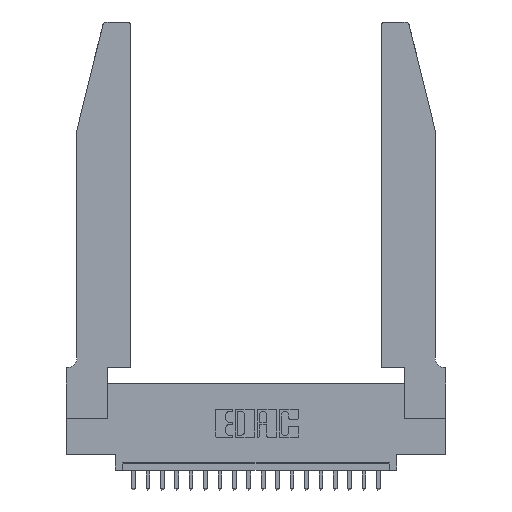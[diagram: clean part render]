
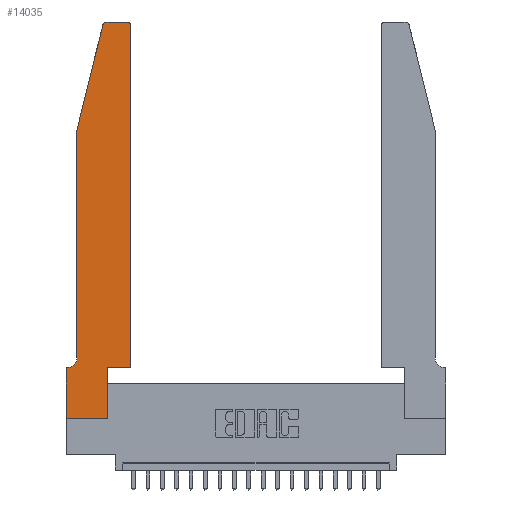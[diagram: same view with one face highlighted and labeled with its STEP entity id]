
A CAD part, top view. The second image highlights one B-rep face of the part: STEP entity #14035.
In plain terms, the highlighted planar face has unit normal (0, 0, 1).
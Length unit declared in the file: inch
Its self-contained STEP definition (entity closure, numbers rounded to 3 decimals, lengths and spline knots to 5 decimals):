
#150 = VERTEX_POINT ( 'NONE', #3158 ) ;
#378 = CARTESIAN_POINT ( 'NONE',  ( 0., 0., 0.37 ) ) ;
#388 = AXIS2_PLACEMENT_3D ( 'NONE', #6410, #19944, #12965 ) ;
#404 = VERTEX_POINT ( 'NONE', #1199 ) ;
#863 = DIRECTION ( 'NONE',  ( -1., 0., 0. ) ) ;
#1165 = LINE ( 'NONE', #7413, #15351 ) ;
#1199 = CARTESIAN_POINT ( 'NONE',  ( 0.25487, 2.72718, 0.37 ) ) ;
#1498 = VERTEX_POINT ( 'NONE', #12572 ) ;
#1550 = VERTEX_POINT ( 'NONE', #11248 ) ;
#1951 = EDGE_CURVE ( 'NONE', #150, #15944, #6328, .T. ) ;
#2256 = EDGE_CURVE ( 'NONE', #1498, #12166, #5822, .T. ) ;
#2539 = CIRCLE ( 'NONE', #16249, 0.03 ) ;
#2664 = DIRECTION ( 'NONE',  ( -1., 0., 0. ) ) ;
#3134 = CARTESIAN_POINT ( 'NONE',  ( 0.2865, 0., 0.37 ) ) ;
#3158 = CARTESIAN_POINT ( 'NONE',  ( 0.0755, 0.42, 0.37 ) ) ;
#3161 = CARTESIAN_POINT ( 'NONE',  ( 0.4505, 0.35, 0.37 ) ) ;
#3423 = DIRECTION ( 'NONE',  ( 0., 1., 0. ) ) ;
#3973 = DIRECTION ( 'NONE',  ( 0., 1., 0. ) ) ;
#4197 = VERTEX_POINT ( 'NONE', #13778 ) ;
#4303 = PLANE ( 'NONE',  #16320 ) ;
#4590 = VERTEX_POINT ( 'NONE', #8246 ) ;
#4596 = EDGE_CURVE ( 'NONE', #1550, #150, #16004, .T. ) ;
#4600 = LINE ( 'NONE', #3161, #20639 ) ;
#4696 = EDGE_LOOP ( 'NONE', ( #13682, #17615, #16482, #18126, #14326, #13669, #9880, #19805, #5662, #19919, #7811, #12443 ) ) ;
#5203 = LINE ( 'NONE', #5921, #19636 ) ;
#5378 = DIRECTION ( 'NONE',  ( 1., 0., 0. ) ) ;
#5662 = ORIENTED_EDGE ( 'NONE', *, *, #7696, .T. ) ;
#5822 = LINE ( 'NONE', #18886, #13185 ) ;
#5921 = CARTESIAN_POINT ( 'NONE',  ( 0.2605, 2.75, 0.37 ) ) ;
#6328 = CIRCLE ( 'NONE', #17832, 0.07 ) ;
#6410 = CARTESIAN_POINT ( 'NONE',  ( 0.284, 2.72, 0.37 ) ) ;
#6680 = VECTOR ( 'NONE', #3973, 39.37008 ) ;
#6788 = DIRECTION ( 'NONE',  ( 0., -1., 0. ) ) ;
#7171 = CARTESIAN_POINT ( 'NONE',  ( 0.4505, 0.35, 0.37 ) ) ;
#7272 = EDGE_CURVE ( 'NONE', #20779, #11202, #4600, .T. ) ;
#7413 = CARTESIAN_POINT ( 'NONE',  ( 0.0755, 0.35, 0.37 ) ) ;
#7421 = DIRECTION ( 'NONE',  ( 0., 0., -1. ) ) ;
#7562 = EDGE_CURVE ( 'NONE', #11202, #4197, #13277, .T. ) ;
#7578 = DIRECTION ( 'NONE',  ( 0., 0., 1. ) ) ;
#7696 = EDGE_CURVE ( 'NONE', #10893, #20779, #12731, .T. ) ;
#7788 = EDGE_CURVE ( 'NONE', #4590, #404, #11410, .T. ) ;
#7811 = ORIENTED_EDGE ( 'NONE', *, *, #7562, .T. ) ;
#8246 = CARTESIAN_POINT ( 'NONE',  ( 0.284, 2.75, 0.37 ) ) ;
#8333 = CARTESIAN_POINT ( 'NONE',  ( 0.0755, 2., 0.37 ) ) ;
#9270 = DIRECTION ( 'NONE',  ( 1., 0., 0. ) ) ;
#9790 = LINE ( 'NONE', #16785, #16121 ) ;
#9880 = ORIENTED_EDGE ( 'NONE', *, *, #2256, .T. ) ;
#9930 = VECTOR ( 'NONE', #6788, 39.37008 ) ;
#10200 = EDGE_CURVE ( 'NONE', #4197, #20260, #2539, .T. ) ;
#10612 = VECTOR ( 'NONE', #3423, 39.37008 ) ;
#10893 = VERTEX_POINT ( 'NONE', #3134 ) ;
#11077 = DIRECTION ( 'NONE',  ( -1., 0., 0. ) ) ;
#11202 = VERTEX_POINT ( 'NONE', #7171 ) ;
#11248 = CARTESIAN_POINT ( 'NONE',  ( 0.0755, 2., 0.37 ) ) ;
#11309 = EDGE_CURVE ( 'NONE', #20260, #4590, #5203, .T. ) ;
#11410 = CIRCLE ( 'NONE', #388, 0.03 ) ;
#12074 = DIRECTION ( 'NONE',  ( 0., 0., 1. ) ) ;
#12166 = VERTEX_POINT ( 'NONE', #378 ) ;
#12443 = ORIENTED_EDGE ( 'NONE', *, *, #10200, .T. ) ;
#12572 = CARTESIAN_POINT ( 'NONE',  ( 0., 0.35, 0.37 ) ) ;
#12582 = EDGE_CURVE ( 'NONE', #404, #1550, #20129, .T. ) ;
#12731 = LINE ( 'NONE', #13953, #6680 ) ;
#12965 = DIRECTION ( 'NONE',  ( 1., 0., 0. ) ) ;
#13081 = CARTESIAN_POINT ( 'NONE',  ( 0.0755, 2., 0.37 ) ) ;
#13185 = VECTOR ( 'NONE', #15936, 39.37008 ) ;
#13256 = FACE_OUTER_BOUND ( 'NONE', #4696, .T. ) ;
#13277 = LINE ( 'NONE', #13437, #10612 ) ;
#13437 = CARTESIAN_POINT ( 'NONE',  ( 0.4505, 0.35, 0.37 ) ) ;
#13669 = ORIENTED_EDGE ( 'NONE', *, *, #17883, .T. ) ;
#13682 = ORIENTED_EDGE ( 'NONE', *, *, #11309, .T. ) ;
#13778 = CARTESIAN_POINT ( 'NONE',  ( 0.4505, 2.72, 0.37 ) ) ;
#13953 = CARTESIAN_POINT ( 'NONE',  ( 0.2865, 0.35, 0.37 ) ) ;
#14035 = ADVANCED_FACE ( 'NONE', ( #13256 ), #4303, .T. ) ;
#14134 = CARTESIAN_POINT ( 'NONE',  ( 0.0055, 0.42, 0.37 ) ) ;
#14292 = EDGE_CURVE ( 'NONE', #12166, #10893, #9790, .T. ) ;
#14326 = ORIENTED_EDGE ( 'NONE', *, *, #1951, .T. ) ;
#15351 = VECTOR ( 'NONE', #11077, 39.37008 ) ;
#15908 = CARTESIAN_POINT ( 'NONE',  ( 0., 0.35, 0.37 ) ) ;
#15936 = DIRECTION ( 'NONE',  ( 0., -1., 0. ) ) ;
#15944 = VERTEX_POINT ( 'NONE', #18100 ) ;
#16004 = LINE ( 'NONE', #8333, #9930 ) ;
#16121 = VECTOR ( 'NONE', #21512, 39.37008 ) ;
#16249 = AXIS2_PLACEMENT_3D ( 'NONE', #20429, #12074, #5378 ) ;
#16320 = AXIS2_PLACEMENT_3D ( 'NONE', #15908, #7578, #9270 ) ;
#16482 = ORIENTED_EDGE ( 'NONE', *, *, #12582, .T. ) ;
#16689 = DIRECTION ( 'NONE',  ( -0.239, -0.971, 0. ) ) ;
#16785 = CARTESIAN_POINT ( 'NONE',  ( 0., 0., 0.37 ) ) ;
#16979 = VECTOR ( 'NONE', #16689, 39.37008 ) ;
#17163 = CARTESIAN_POINT ( 'NONE',  ( 0.2865, 0.35, 0.37 ) ) ;
#17615 = ORIENTED_EDGE ( 'NONE', *, *, #7788, .T. ) ;
#17832 = AXIS2_PLACEMENT_3D ( 'NONE', #14134, #7421, #863 ) ;
#17883 = EDGE_CURVE ( 'NONE', #15944, #1498, #1165, .T. ) ;
#18100 = CARTESIAN_POINT ( 'NONE',  ( 0.0055, 0.35, 0.37 ) ) ;
#18126 = ORIENTED_EDGE ( 'NONE', *, *, #4596, .T. ) ;
#18886 = CARTESIAN_POINT ( 'NONE',  ( 0., 0., 0.37 ) ) ;
#19636 = VECTOR ( 'NONE', #2664, 39.37008 ) ;
#19805 = ORIENTED_EDGE ( 'NONE', *, *, #14292, .T. ) ;
#19919 = ORIENTED_EDGE ( 'NONE', *, *, #7272, .T. ) ;
#19944 = DIRECTION ( 'NONE',  ( 0., 0., 1. ) ) ;
#20129 = LINE ( 'NONE', #13081, #16979 ) ;
#20260 = VERTEX_POINT ( 'NONE', #20302 ) ;
#20302 = CARTESIAN_POINT ( 'NONE',  ( 0.4205, 2.75, 0.37 ) ) ;
#20376 = DIRECTION ( 'NONE',  ( 1., 0., 0. ) ) ;
#20429 = CARTESIAN_POINT ( 'NONE',  ( 0.4205, 2.72, 0.37 ) ) ;
#20639 = VECTOR ( 'NONE', #20376, 39.37008 ) ;
#20779 = VERTEX_POINT ( 'NONE', #17163 ) ;
#21512 = DIRECTION ( 'NONE',  ( 1., 0., 0. ) ) ;
